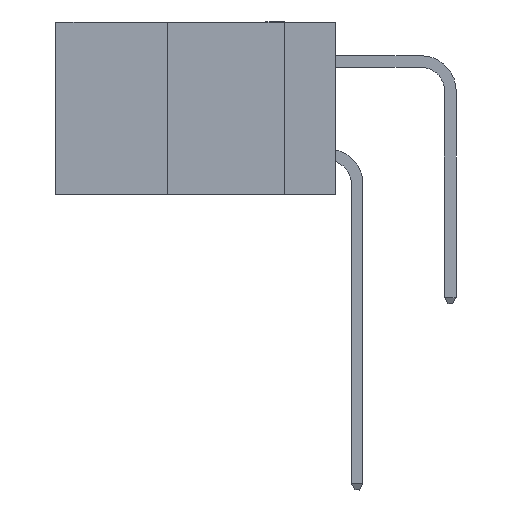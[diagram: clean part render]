
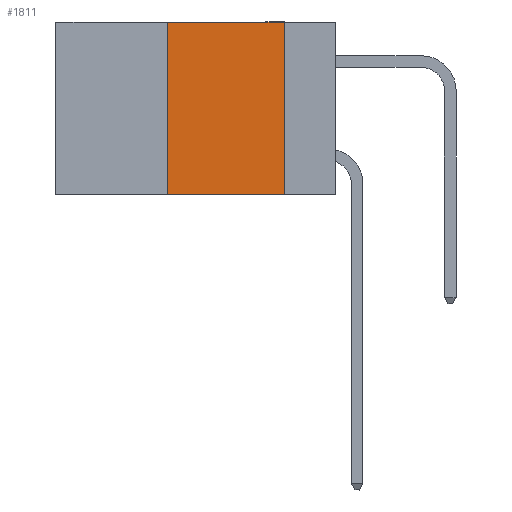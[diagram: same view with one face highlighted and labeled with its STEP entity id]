
A CAD part, left-side view. The second image highlights one B-rep face of the part: STEP entity #1811.
In plain terms, the highlighted planar face has unit normal (-1, 0, 0).
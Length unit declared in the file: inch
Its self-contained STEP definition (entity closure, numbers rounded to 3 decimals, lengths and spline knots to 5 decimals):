
#1811 = ADVANCED_FACE ( 'NONE', ( #7262 ), #14112, .F. ) ;
#2399 = LINE ( 'NONE', #15768, #2521 ) ;
#2521 = VECTOR ( 'NONE', #21147, 39.37008 ) ;
#3307 = CARTESIAN_POINT ( 'NONE',  ( 0., 0.6, -0.37 ) ) ;
#3442 = ORIENTED_EDGE ( 'NONE', *, *, #22176, .F. ) ;
#3729 = AXIS2_PLACEMENT_3D ( 'NONE', #7594, #20962, #12427 ) ;
#3797 = EDGE_CURVE ( 'NONE', #12890, #17806, #6675, .T. ) ;
#3958 = DIRECTION ( 'NONE',  ( 0., 0., -1. ) ) ;
#5096 = DIRECTION ( 'NONE',  ( 0., 0., 1. ) ) ;
#6675 = LINE ( 'NONE', #13736, #16832 ) ;
#7002 = LINE ( 'NONE', #10797, #17000 ) ;
#7262 = FACE_OUTER_BOUND ( 'NONE', #11335, .T. ) ;
#7594 = CARTESIAN_POINT ( 'NONE',  ( 0., 0.6, 0. ) ) ;
#8032 = CARTESIAN_POINT ( 'NONE',  ( 0., 0.11, 0. ) ) ;
#8333 = VERTEX_POINT ( 'NONE', #8032 ) ;
#10006 = CARTESIAN_POINT ( 'NONE',  ( 0., 0.11, -0.37 ) ) ;
#10797 = CARTESIAN_POINT ( 'NONE',  ( 0., 0.11, 0. ) ) ;
#11335 = EDGE_LOOP ( 'NONE', ( #3442, #16424, #16496, #17997 ) ) ;
#12427 = DIRECTION ( 'NONE',  ( 0., 0., -1. ) ) ;
#12890 = VERTEX_POINT ( 'NONE', #20611 ) ;
#13736 = CARTESIAN_POINT ( 'NONE',  ( 0., 0.36, 0. ) ) ;
#14112 = PLANE ( 'NONE',  #3729 ) ;
#15110 = VECTOR ( 'NONE', #17023, 39.37008 ) ;
#15547 = CARTESIAN_POINT ( 'NONE',  ( 0., 0.36, 0. ) ) ;
#15768 = CARTESIAN_POINT ( 'NONE',  ( 0., 0.6, 0. ) ) ;
#15957 = EDGE_CURVE ( 'NONE', #17806, #8333, #2399, .T. ) ;
#16424 = ORIENTED_EDGE ( 'NONE', *, *, #15957, .F. ) ;
#16496 = ORIENTED_EDGE ( 'NONE', *, *, #3797, .F. ) ;
#16832 = VECTOR ( 'NONE', #5096, 39.37008 ) ;
#17000 = VECTOR ( 'NONE', #3958, 39.37008 ) ;
#17023 = DIRECTION ( 'NONE',  ( 0., -1., 0. ) ) ;
#17720 = EDGE_CURVE ( 'NONE', #12890, #18105, #21938, .T. ) ;
#17806 = VERTEX_POINT ( 'NONE', #15547 ) ;
#17997 = ORIENTED_EDGE ( 'NONE', *, *, #17720, .T. ) ;
#18105 = VERTEX_POINT ( 'NONE', #10006 ) ;
#20611 = CARTESIAN_POINT ( 'NONE',  ( 0., 0.36, -0.37 ) ) ;
#20962 = DIRECTION ( 'NONE',  ( 1., 0., 0. ) ) ;
#21147 = DIRECTION ( 'NONE',  ( 0., -1., 0. ) ) ;
#21938 = LINE ( 'NONE', #3307, #15110 ) ;
#22176 = EDGE_CURVE ( 'NONE', #8333, #18105, #7002, .T. ) ;
